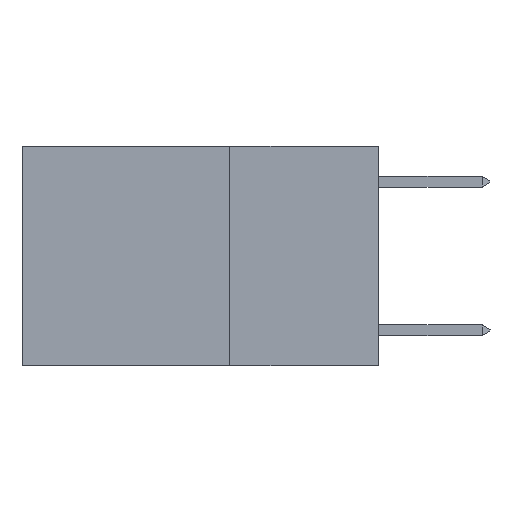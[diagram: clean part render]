
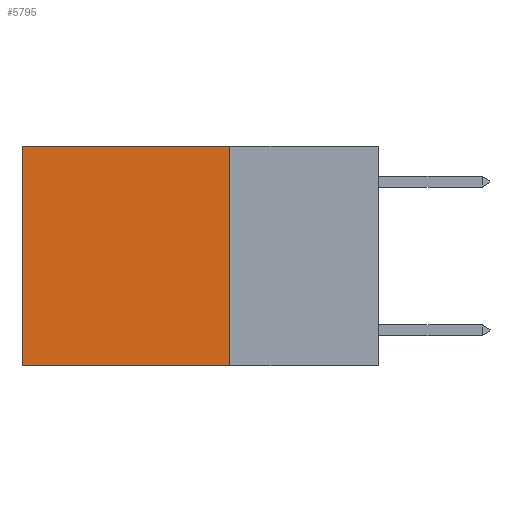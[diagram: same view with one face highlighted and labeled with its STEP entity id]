
A CAD part, left-side view. The second image highlights one B-rep face of the part: STEP entity #5795.
In plain terms, the highlighted planar face has unit normal (-1, 0, 0).
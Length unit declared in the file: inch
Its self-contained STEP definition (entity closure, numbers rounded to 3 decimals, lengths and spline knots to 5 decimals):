
#627 = CARTESIAN_POINT ( 'NONE',  ( 0.2625, 0.6, -0.37 ) ) ;
#838 = CARTESIAN_POINT ( 'NONE',  ( 0.2625, 0.6, 0. ) ) ;
#2903 = EDGE_CURVE ( 'NONE', #14113, #4546, #14857, .T. ) ;
#3180 = CARTESIAN_POINT ( 'NONE',  ( 0.2625, 0.6, 0. ) ) ;
#3850 = VERTEX_POINT ( 'NONE', #838 ) ;
#4217 = DIRECTION ( 'NONE',  ( 0., 0., -1. ) ) ;
#4546 = VERTEX_POINT ( 'NONE', #17089 ) ;
#4651 = CARTESIAN_POINT ( 'NONE',  ( 0.2625, 0.25, 0. ) ) ;
#4830 = DIRECTION ( 'NONE',  ( 0., 0., -1. ) ) ;
#5395 = LINE ( 'NONE', #8547, #5562 ) ;
#5562 = VECTOR ( 'NONE', #8517, 39.37008 ) ;
#5795 = ADVANCED_FACE ( 'NONE', ( #13179 ), #9831, .F. ) ;
#8019 = DIRECTION ( 'NONE',  ( 0., 0., -1. ) ) ;
#8517 = DIRECTION ( 'NONE',  ( 0., 1., 0. ) ) ;
#8547 = CARTESIAN_POINT ( 'NONE',  ( 0.2625, 0.25, 0. ) ) ;
#8598 = DIRECTION ( 'NONE',  ( 1., 0., 0. ) ) ;
#8760 = CARTESIAN_POINT ( 'NONE',  ( 0.2625, 0.25, 0. ) ) ;
#9831 = PLANE ( 'NONE',  #13978 ) ;
#11146 = EDGE_CURVE ( 'NONE', #14113, #3850, #5395, .T. ) ;
#11207 = ORIENTED_EDGE ( 'NONE', *, *, #2903, .F. ) ;
#12309 = EDGE_CURVE ( 'NONE', #4546, #21134, #15327, .T. ) ;
#13179 = FACE_OUTER_BOUND ( 'NONE', #15383, .T. ) ;
#13183 = CARTESIAN_POINT ( 'NONE',  ( 0.2625, 0.25, 0. ) ) ;
#13978 = AXIS2_PLACEMENT_3D ( 'NONE', #8760, #8598, #8019 ) ;
#14113 = VERTEX_POINT ( 'NONE', #13183 ) ;
#14209 = ORIENTED_EDGE ( 'NONE', *, *, #12309, .F. ) ;
#14581 = VECTOR ( 'NONE', #4217, 39.37008 ) ;
#14857 = LINE ( 'NONE', #4651, #14581 ) ;
#15288 = VECTOR ( 'NONE', #16901, 39.37008 ) ;
#15327 = LINE ( 'NONE', #17123, #15288 ) ;
#15383 = EDGE_LOOP ( 'NONE', ( #20918, #14209, #11207, #16102 ) ) ;
#16102 = ORIENTED_EDGE ( 'NONE', *, *, #11146, .T. ) ;
#16901 = DIRECTION ( 'NONE',  ( 0., 1., 0. ) ) ;
#16977 = VECTOR ( 'NONE', #4830, 39.37008 ) ;
#17060 = LINE ( 'NONE', #3180, #16977 ) ;
#17089 = CARTESIAN_POINT ( 'NONE',  ( 0.2625, 0.25, -0.37 ) ) ;
#17123 = CARTESIAN_POINT ( 'NONE',  ( 0.2625, 0.25, -0.37 ) ) ;
#18599 = EDGE_CURVE ( 'NONE', #3850, #21134, #17060, .T. ) ;
#20918 = ORIENTED_EDGE ( 'NONE', *, *, #18599, .T. ) ;
#21134 = VERTEX_POINT ( 'NONE', #627 ) ;
